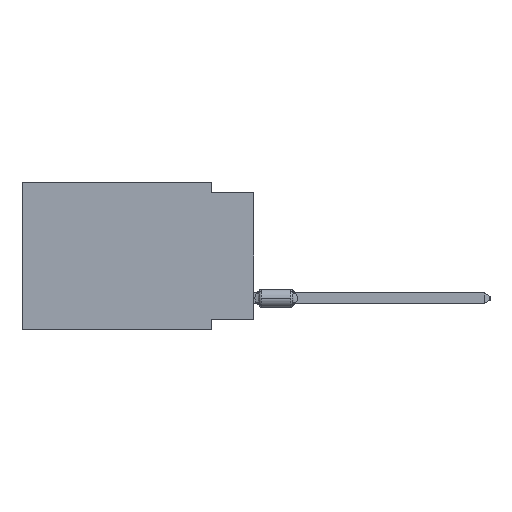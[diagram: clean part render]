
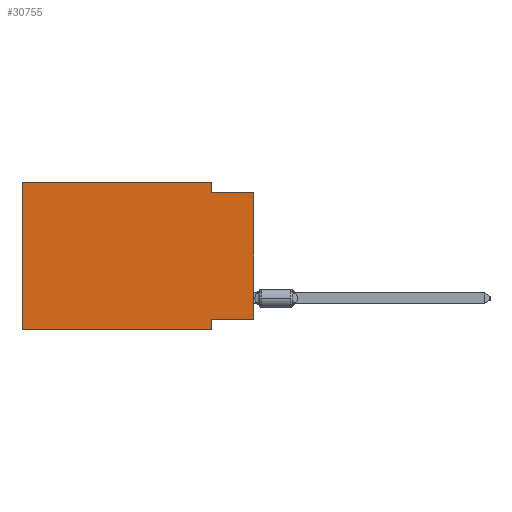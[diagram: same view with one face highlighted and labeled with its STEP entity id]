
A CAD part, left-side view. The second image highlights one B-rep face of the part: STEP entity #30755.
In plain terms, the highlighted planar face has unit normal (-1, 0, 0).
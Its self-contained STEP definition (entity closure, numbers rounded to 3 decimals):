
#1567 = EDGE_CURVE ( 'NONE', #43206, #20188, #37563, .T. ) ;
#2557 = DIRECTION ( 'NONE',  ( 0., -1., 0. ) ) ;
#3961 = CARTESIAN_POINT ( 'NONE',  ( 0., 13.97, -8.89 ) ) ;
#4474 = ORIENTED_EDGE ( 'NONE', *, *, #1567, .F. ) ;
#5164 = DIRECTION ( 'NONE',  ( 0., 0., -1. ) ) ;
#5225 = DIRECTION ( 'NONE',  ( 0., 0., 1. ) ) ;
#5438 = VERTEX_POINT ( 'NONE', #21142 ) ;
#5742 = LINE ( 'NONE', #35005, #10635 ) ;
#6236 = CARTESIAN_POINT ( 'NONE',  ( 0., 2.54, 0. ) ) ;
#6549 = ORIENTED_EDGE ( 'NONE', *, *, #47132, .T. ) ;
#7660 = CARTESIAN_POINT ( 'NONE',  ( 0., 0., -0.635 ) ) ;
#8833 = CARTESIAN_POINT ( 'NONE',  ( 0., 13.97, 0. ) ) ;
#9619 = LINE ( 'NONE', #38659, #47404 ) ;
#10265 = ORIENTED_EDGE ( 'NONE', *, *, #46992, .T. ) ;
#10635 = VECTOR ( 'NONE', #30916, 1000. ) ;
#11356 = CARTESIAN_POINT ( 'NONE',  ( 0., 13.97, 0. ) ) ;
#11901 = CARTESIAN_POINT ( 'NONE',  ( 0., 2.54, -8.89 ) ) ;
#12838 = VECTOR ( 'NONE', #5225, 1000. ) ;
#13915 = VERTEX_POINT ( 'NONE', #38703 ) ;
#16770 = VECTOR ( 'NONE', #31873, 1000. ) ;
#17120 = CARTESIAN_POINT ( 'NONE',  ( 0., 13.97, -8.89 ) ) ;
#19987 = AXIS2_PLACEMENT_3D ( 'NONE', #11356, #26212, #36555 ) ;
#19998 = VECTOR ( 'NONE', #24680, 1000. ) ;
#20188 = VERTEX_POINT ( 'NONE', #32365 ) ;
#20197 = EDGE_CURVE ( 'NONE', #31236, #46554, #20857, .T. ) ;
#20857 = LINE ( 'NONE', #6236, #19998 ) ;
#21142 = CARTESIAN_POINT ( 'NONE',  ( 0., 0., -8.255 ) ) ;
#21662 = ORIENTED_EDGE ( 'NONE', *, *, #20197, .F. ) ;
#23801 = CARTESIAN_POINT ( 'NONE',  ( 0., 0., -8.255 ) ) ;
#24005 = CARTESIAN_POINT ( 'NONE',  ( 0., 2.54, -0.635 ) ) ;
#24680 = DIRECTION ( 'NONE',  ( 0., 0., -1. ) ) ;
#26212 = DIRECTION ( 'NONE',  ( 1., 0., 0. ) ) ;
#26865 = ORIENTED_EDGE ( 'NONE', *, *, #32746, .F. ) ;
#27949 = EDGE_CURVE ( 'NONE', #43104, #13915, #41716, .T. ) ;
#28822 = ORIENTED_EDGE ( 'NONE', *, *, #29799, .F. ) ;
#29799 = EDGE_CURVE ( 'NONE', #5438, #43206, #42303, .T. ) ;
#30755 = ADVANCED_FACE ( 'NONE', ( #39953 ), #44229, .F. ) ;
#30916 = DIRECTION ( 'NONE',  ( 0., 0., 1. ) ) ;
#31137 = EDGE_LOOP ( 'NONE', ( #10265, #44925, #21662, #26865, #33435, #6549, #4474, #28822 ) ) ;
#31236 = VERTEX_POINT ( 'NONE', #41528 ) ;
#31588 = CARTESIAN_POINT ( 'NONE',  ( 0., 13.97, 0. ) ) ;
#31873 = DIRECTION ( 'NONE',  ( 0., -1., 0. ) ) ;
#32365 = CARTESIAN_POINT ( 'NONE',  ( 0., 2.54, -8.89 ) ) ;
#32746 = EDGE_CURVE ( 'NONE', #13915, #31236, #39281, .T. ) ;
#33435 = ORIENTED_EDGE ( 'NONE', *, *, #27949, .F. ) ;
#35005 = CARTESIAN_POINT ( 'NONE',  ( 0., 0., 0. ) ) ;
#36555 = DIRECTION ( 'NONE',  ( 0., 0., -1. ) ) ;
#36979 = CARTESIAN_POINT ( 'NONE',  ( 0., 2.54, -8.255 ) ) ;
#37563 = LINE ( 'NONE', #11901, #41570 ) ;
#38309 = VECTOR ( 'NONE', #38686, 1000. ) ;
#38659 = CARTESIAN_POINT ( 'NONE',  ( 0., 0., -0.635 ) ) ;
#38686 = DIRECTION ( 'NONE',  ( 0., 1., 0. ) ) ;
#38703 = CARTESIAN_POINT ( 'NONE',  ( 0., 13.97, 0. ) ) ;
#38895 = DIRECTION ( 'NONE',  ( 0., -1., 0. ) ) ;
#39281 = LINE ( 'NONE', #31588, #43548 ) ;
#39953 = FACE_OUTER_BOUND ( 'NONE', #31137, .T. ) ;
#41528 = CARTESIAN_POINT ( 'NONE',  ( 0., 2.54, 0. ) ) ;
#41570 = VECTOR ( 'NONE', #5164, 1000. ) ;
#41716 = LINE ( 'NONE', #8833, #12838 ) ;
#42303 = LINE ( 'NONE', #23801, #38309 ) ;
#43104 = VERTEX_POINT ( 'NONE', #17120 ) ;
#43206 = VERTEX_POINT ( 'NONE', #36979 ) ;
#43548 = VECTOR ( 'NONE', #2557, 1000. ) ;
#43829 = VERTEX_POINT ( 'NONE', #7660 ) ;
#44229 = PLANE ( 'NONE',  #19987 ) ;
#44925 = ORIENTED_EDGE ( 'NONE', *, *, #46600, .F. ) ;
#46535 = LINE ( 'NONE', #3961, #16770 ) ;
#46554 = VERTEX_POINT ( 'NONE', #24005 ) ;
#46600 = EDGE_CURVE ( 'NONE', #46554, #43829, #9619, .T. ) ;
#46992 = EDGE_CURVE ( 'NONE', #5438, #43829, #5742, .T. ) ;
#47132 = EDGE_CURVE ( 'NONE', #43104, #20188, #46535, .T. ) ;
#47404 = VECTOR ( 'NONE', #38895, 1000. ) ;
